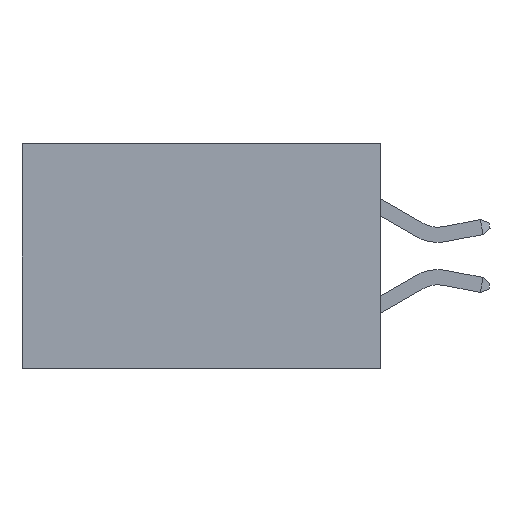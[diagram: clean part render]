
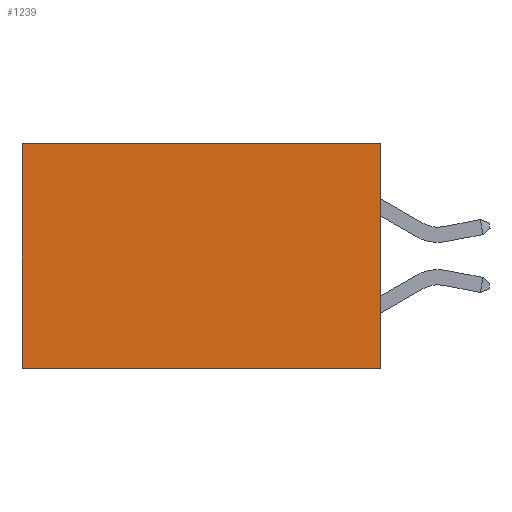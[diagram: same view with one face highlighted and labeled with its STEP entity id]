
A CAD part, left-side view. The second image highlights one B-rep face of the part: STEP entity #1239.
In plain terms, the highlighted planar face has unit normal (-1, 0, 0).
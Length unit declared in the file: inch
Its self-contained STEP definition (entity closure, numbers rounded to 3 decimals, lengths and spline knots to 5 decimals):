
#1239 = ADVANCED_FACE ( 'NONE', ( #20473 ), #2696, .F. ) ;
#1639 = EDGE_CURVE ( 'NONE', #4762, #9553, #26710, .T. ) ;
#2187 = VECTOR ( 'NONE', #19938, 39.37008 ) ;
#2194 = AXIS2_PLACEMENT_3D ( 'NONE', #2660, #14219, #14108 ) ;
#2363 = EDGE_LOOP ( 'NONE', ( #31011, #28987, #13981, #30805 ) ) ;
#2660 = CARTESIAN_POINT ( 'NONE',  ( 0.277, 0., -0.37 ) ) ;
#2696 = PLANE ( 'NONE',  #2194 ) ;
#4762 = VERTEX_POINT ( 'NONE', #18200 ) ;
#5278 = LINE ( 'NONE', #25601, #32889 ) ;
#5438 = VECTOR ( 'NONE', #5705, 39.37008 ) ;
#5705 = DIRECTION ( 'NONE',  ( 0., 1., 0. ) ) ;
#6025 = VERTEX_POINT ( 'NONE', #32980 ) ;
#6474 = EDGE_CURVE ( 'NONE', #4762, #22774, #5278, .T. ) ;
#8596 = EDGE_CURVE ( 'NONE', #9553, #6025, #9338, .T. ) ;
#9338 = LINE ( 'NONE', #19818, #2187 ) ;
#9553 = VERTEX_POINT ( 'NONE', #23264 ) ;
#13981 = ORIENTED_EDGE ( 'NONE', *, *, #6474, .F. ) ;
#14108 = DIRECTION ( 'NONE',  ( 0., 0., -1. ) ) ;
#14219 = DIRECTION ( 'NONE',  ( 1., 0., 0. ) ) ;
#18200 = CARTESIAN_POINT ( 'NONE',  ( 0.277, 0., 0. ) ) ;
#18868 = LINE ( 'NONE', #21790, #5438 ) ;
#19783 = EDGE_CURVE ( 'NONE', #22774, #6025, #18868, .T. ) ;
#19818 = CARTESIAN_POINT ( 'NONE',  ( 0.277, 0.59, -0.37 ) ) ;
#19938 = DIRECTION ( 'NONE',  ( 0., 0., -1. ) ) ;
#20473 = FACE_OUTER_BOUND ( 'NONE', #2363, .T. ) ;
#21790 = CARTESIAN_POINT ( 'NONE',  ( 0.277, 0., -0.37 ) ) ;
#22774 = VERTEX_POINT ( 'NONE', #31352 ) ;
#23264 = CARTESIAN_POINT ( 'NONE',  ( 0.277, 0.59, 0. ) ) ;
#25380 = DIRECTION ( 'NONE',  ( 0., 0., -1. ) ) ;
#25601 = CARTESIAN_POINT ( 'NONE',  ( 0.277, 0., -0.37 ) ) ;
#26474 = CARTESIAN_POINT ( 'NONE',  ( 0.277, 0., 0. ) ) ;
#26710 = LINE ( 'NONE', #26474, #33744 ) ;
#27151 = DIRECTION ( 'NONE',  ( 0., 1., 0. ) ) ;
#28987 = ORIENTED_EDGE ( 'NONE', *, *, #19783, .F. ) ;
#30805 = ORIENTED_EDGE ( 'NONE', *, *, #1639, .T. ) ;
#31011 = ORIENTED_EDGE ( 'NONE', *, *, #8596, .T. ) ;
#31352 = CARTESIAN_POINT ( 'NONE',  ( 0.277, 0., -0.37 ) ) ;
#32889 = VECTOR ( 'NONE', #25380, 39.37008 ) ;
#32980 = CARTESIAN_POINT ( 'NONE',  ( 0.277, 0.59, -0.37 ) ) ;
#33744 = VECTOR ( 'NONE', #27151, 39.37008 ) ;
